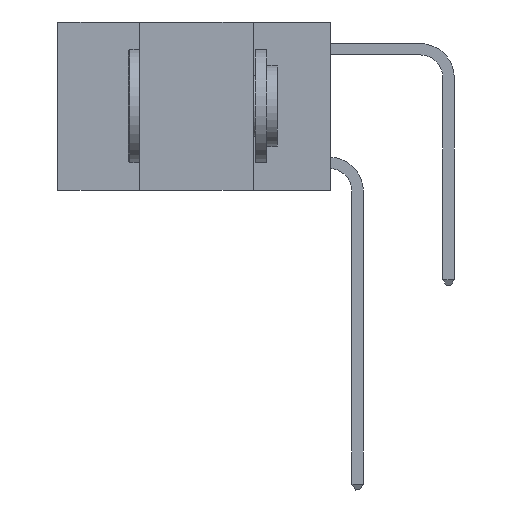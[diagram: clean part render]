
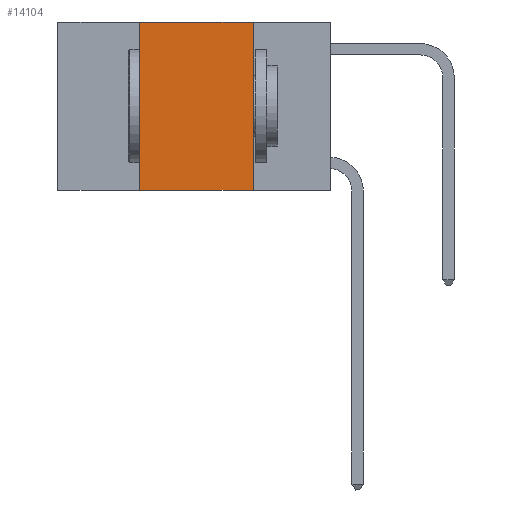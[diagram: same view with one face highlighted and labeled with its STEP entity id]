
A CAD part, left-side view. The second image highlights one B-rep face of the part: STEP entity #14104.
In plain terms, the highlighted planar face has unit normal (-1, 0, 0).
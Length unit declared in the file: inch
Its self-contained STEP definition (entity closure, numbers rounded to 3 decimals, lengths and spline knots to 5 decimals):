
#466 = VECTOR ( 'NONE', #12758, 39.37008 ) ;
#542 = PLANE ( 'NONE',  #641 ) ;
#641 = AXIS2_PLACEMENT_3D ( 'NONE', #11841, #7006, #17115 ) ;
#2151 = CARTESIAN_POINT ( 'NONE',  ( 0., 0.17, 0. ) ) ;
#2490 = VERTEX_POINT ( 'NONE', #20779 ) ;
#2802 = ORIENTED_EDGE ( 'NONE', *, *, #21275, .F. ) ;
#3358 = VECTOR ( 'NONE', #11040, 39.37008 ) ;
#4145 = DIRECTION ( 'NONE',  ( 0., 0., 1. ) ) ;
#4209 = CARTESIAN_POINT ( 'NONE',  ( 0., 0.6, -0.37 ) ) ;
#4427 = LINE ( 'NONE', #4209, #3358 ) ;
#4995 = CARTESIAN_POINT ( 'NONE',  ( 0., 0.42, -0.37 ) ) ;
#5676 = LINE ( 'NONE', #17443, #6824 ) ;
#6167 = VERTEX_POINT ( 'NONE', #15517 ) ;
#6824 = VECTOR ( 'NONE', #4145, 39.37008 ) ;
#7006 = DIRECTION ( 'NONE',  ( 1., 0., 0. ) ) ;
#7570 = VECTOR ( 'NONE', #8777, 39.37008 ) ;
#7828 = ORIENTED_EDGE ( 'NONE', *, *, #17116, .F. ) ;
#8777 = DIRECTION ( 'NONE',  ( 0., 0., -1. ) ) ;
#10880 = CARTESIAN_POINT ( 'NONE',  ( 0., 0.17, -0.37 ) ) ;
#11040 = DIRECTION ( 'NONE',  ( 0., -1., 0. ) ) ;
#11195 = LINE ( 'NONE', #14523, #466 ) ;
#11508 = VERTEX_POINT ( 'NONE', #10880 ) ;
#11729 = VERTEX_POINT ( 'NONE', #4995 ) ;
#11841 = CARTESIAN_POINT ( 'NONE',  ( 0., 0.6, 0. ) ) ;
#11850 = LINE ( 'NONE', #2151, #7570 ) ;
#11991 = ORIENTED_EDGE ( 'NONE', *, *, #12466, .T. ) ;
#12466 = EDGE_CURVE ( 'NONE', #11729, #11508, #4427, .T. ) ;
#12758 = DIRECTION ( 'NONE',  ( 0., -1., 0. ) ) ;
#14104 = ADVANCED_FACE ( 'NONE', ( #15357 ), #542, .F. ) ;
#14523 = CARTESIAN_POINT ( 'NONE',  ( 0., 0.6, 0. ) ) ;
#15357 = FACE_OUTER_BOUND ( 'NONE', #17896, .T. ) ;
#15517 = CARTESIAN_POINT ( 'NONE',  ( 0., 0.17, 0. ) ) ;
#17115 = DIRECTION ( 'NONE',  ( 0., 0., -1. ) ) ;
#17116 = EDGE_CURVE ( 'NONE', #2490, #6167, #11195, .T. ) ;
#17443 = CARTESIAN_POINT ( 'NONE',  ( 0., 0.42, 0. ) ) ;
#17896 = EDGE_LOOP ( 'NONE', ( #2802, #7828, #18923, #11991 ) ) ;
#18444 = EDGE_CURVE ( 'NONE', #11729, #2490, #5676, .T. ) ;
#18923 = ORIENTED_EDGE ( 'NONE', *, *, #18444, .F. ) ;
#20779 = CARTESIAN_POINT ( 'NONE',  ( 0., 0.42, 0. ) ) ;
#21275 = EDGE_CURVE ( 'NONE', #6167, #11508, #11850, .T. ) ;
